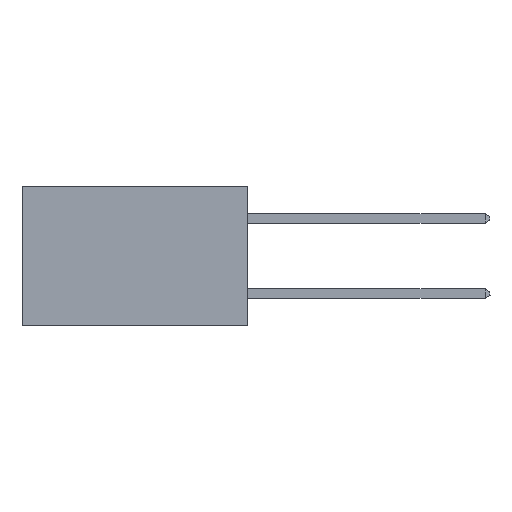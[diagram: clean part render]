
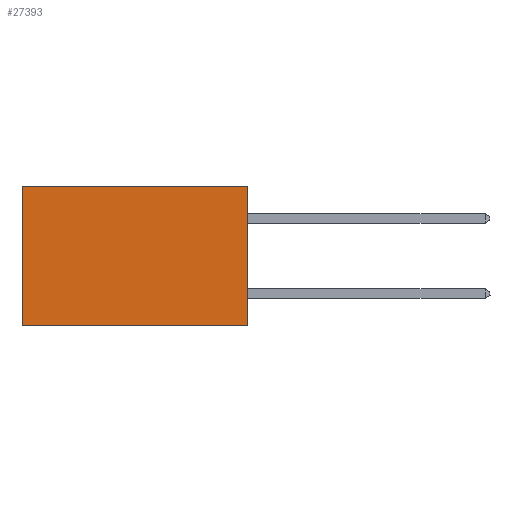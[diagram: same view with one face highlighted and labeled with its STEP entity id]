
A CAD part, left-side view. The second image highlights one B-rep face of the part: STEP entity #27393.
In plain terms, the highlighted planar face has unit normal (-1, 0, 0).
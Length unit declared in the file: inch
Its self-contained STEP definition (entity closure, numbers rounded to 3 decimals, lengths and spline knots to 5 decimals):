
#949 = AXIS2_PLACEMENT_3D ( 'NONE', #20431, #2049, #23028 ) ;
#1285 = VERTEX_POINT ( 'NONE', #14208 ) ;
#1829 = VECTOR ( 'NONE', #8247, 39.37008 ) ;
#1876 = LINE ( 'NONE', #29068, #14083 ) ;
#2049 = DIRECTION ( 'NONE',  ( 1., 0., 0. ) ) ;
#2832 = CARTESIAN_POINT ( 'NONE',  ( 0.298, 0., 0. ) ) ;
#5426 = EDGE_CURVE ( 'NONE', #22042, #1285, #1876, .T. ) ;
#5774 = ORIENTED_EDGE ( 'NONE', *, *, #19400, .T. ) ;
#6655 = CARTESIAN_POINT ( 'NONE',  ( 0.298, 0.6, -0.37 ) ) ;
#8235 = LINE ( 'NONE', #2832, #10034 ) ;
#8247 = DIRECTION ( 'NONE',  ( 0., 0., -1. ) ) ;
#8575 = CARTESIAN_POINT ( 'NONE',  ( 0.298, 0., 0. ) ) ;
#9440 = ORIENTED_EDGE ( 'NONE', *, *, #18534, .T. ) ;
#9774 = ORIENTED_EDGE ( 'NONE', *, *, #5426, .F. ) ;
#10034 = VECTOR ( 'NONE', #14697, 39.37008 ) ;
#10970 = CARTESIAN_POINT ( 'NONE',  ( 0.298, 0.6, 0. ) ) ;
#11478 = VECTOR ( 'NONE', #25048, 39.37008 ) ;
#11965 = VERTEX_POINT ( 'NONE', #6655 ) ;
#12796 = EDGE_CURVE ( 'NONE', #1285, #11965, #21521, .T. ) ;
#14083 = VECTOR ( 'NONE', #24584, 39.37008 ) ;
#14208 = CARTESIAN_POINT ( 'NONE',  ( 0.298, 0., -0.37 ) ) ;
#14697 = DIRECTION ( 'NONE',  ( 0., 1., 0. ) ) ;
#15827 = PLANE ( 'NONE',  #949 ) ;
#15975 = VERTEX_POINT ( 'NONE', #18712 ) ;
#17693 = ORIENTED_EDGE ( 'NONE', *, *, #12796, .F. ) ;
#18534 = EDGE_CURVE ( 'NONE', #15975, #11965, #25923, .T. ) ;
#18712 = CARTESIAN_POINT ( 'NONE',  ( 0.298, 0.6, 0. ) ) ;
#18919 = FACE_OUTER_BOUND ( 'NONE', #22025, .T. ) ;
#19400 = EDGE_CURVE ( 'NONE', #22042, #15975, #8235, .T. ) ;
#20431 = CARTESIAN_POINT ( 'NONE',  ( 0.298, 0., 0. ) ) ;
#21521 = LINE ( 'NONE', #24952, #11478 ) ;
#22025 = EDGE_LOOP ( 'NONE', ( #9440, #17693, #9774, #5774 ) ) ;
#22042 = VERTEX_POINT ( 'NONE', #8575 ) ;
#23028 = DIRECTION ( 'NONE',  ( 0., 0., -1. ) ) ;
#24584 = DIRECTION ( 'NONE',  ( 0., 0., -1. ) ) ;
#24952 = CARTESIAN_POINT ( 'NONE',  ( 0.298, 0., -0.37 ) ) ;
#25048 = DIRECTION ( 'NONE',  ( 0., 1., 0. ) ) ;
#25923 = LINE ( 'NONE', #10970, #1829 ) ;
#27393 = ADVANCED_FACE ( 'NONE', ( #18919 ), #15827, .F. ) ;
#29068 = CARTESIAN_POINT ( 'NONE',  ( 0.298, 0., 0. ) ) ;
